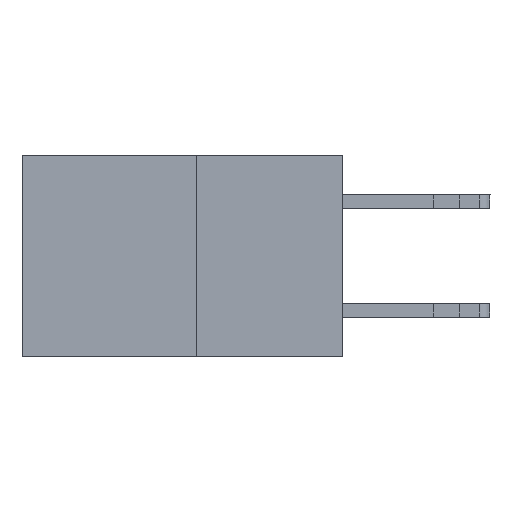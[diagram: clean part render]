
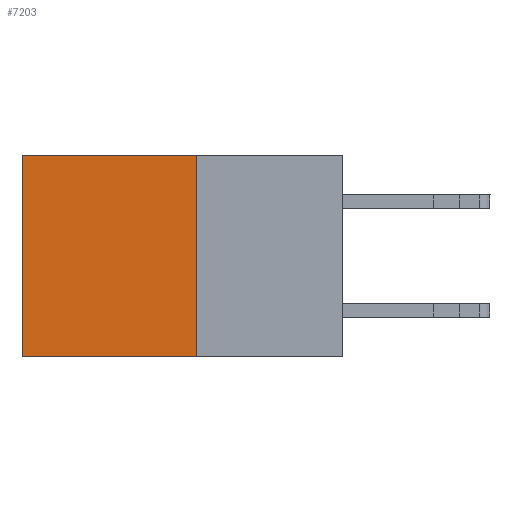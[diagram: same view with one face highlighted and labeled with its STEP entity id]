
A CAD part, left-side view. The second image highlights one B-rep face of the part: STEP entity #7203.
In plain terms, the highlighted planar face has unit normal (-1, 0, 0).
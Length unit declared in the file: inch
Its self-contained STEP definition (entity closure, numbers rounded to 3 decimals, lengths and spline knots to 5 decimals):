
#1 = VECTOR ( 'NONE', #10991, 39.37008 ) ;
#1696 = ORIENTED_EDGE ( 'NONE', *, *, #7137, .T. ) ;
#1968 = FACE_OUTER_BOUND ( 'NONE', #6050, .T. ) ;
#2018 = ORIENTED_EDGE ( 'NONE', *, *, #11326, .F. ) ;
#2251 = VERTEX_POINT ( 'NONE', #2997 ) ;
#2288 = VECTOR ( 'NONE', #6027, 39.37008 ) ;
#2997 = CARTESIAN_POINT ( 'NONE',  ( 0.277, 0.27, -0.37 ) ) ;
#4152 = VERTEX_POINT ( 'NONE', #9362 ) ;
#4315 = CARTESIAN_POINT ( 'NONE',  ( 0.277, 0.27, 0. ) ) ;
#5833 = LINE ( 'NONE', #11762, #2288 ) ;
#6027 = DIRECTION ( 'NONE',  ( 0., 1., 0. ) ) ;
#6050 = EDGE_LOOP ( 'NONE', ( #12384, #2018, #8611, #1696 ) ) ;
#6642 = LINE ( 'NONE', #11061, #1 ) ;
#6974 = EDGE_CURVE ( 'NONE', #4152, #8397, #10709, .T. ) ;
#7137 = EDGE_CURVE ( 'NONE', #12748, #4152, #6642, .T. ) ;
#7203 = ADVANCED_FACE ( 'NONE', ( #1968 ), #9122, .F. ) ;
#7771 = VECTOR ( 'NONE', #11431, 39.37008 ) ;
#8397 = VERTEX_POINT ( 'NONE', #8627 ) ;
#8549 = VECTOR ( 'NONE', #14202, 39.37008 ) ;
#8611 = ORIENTED_EDGE ( 'NONE', *, *, #8908, .F. ) ;
#8627 = CARTESIAN_POINT ( 'NONE',  ( 0.277, 0.59, -0.37 ) ) ;
#8790 = DIRECTION ( 'NONE',  ( 0., 0., -1. ) ) ;
#8835 = DIRECTION ( 'NONE',  ( 1., 0., 0. ) ) ;
#8908 = EDGE_CURVE ( 'NONE', #12748, #2251, #11950, .T. ) ;
#9122 = PLANE ( 'NONE',  #13848 ) ;
#9260 = CARTESIAN_POINT ( 'NONE',  ( 0.277, 0.27, -0.37 ) ) ;
#9362 = CARTESIAN_POINT ( 'NONE',  ( 0.277, 0.59, 0. ) ) ;
#9498 = CARTESIAN_POINT ( 'NONE',  ( 0.277, 0.27, -0.37 ) ) ;
#10709 = LINE ( 'NONE', #12743, #7771 ) ;
#10991 = DIRECTION ( 'NONE',  ( 0., 1., 0. ) ) ;
#11061 = CARTESIAN_POINT ( 'NONE',  ( 0.277, 0.27, 0. ) ) ;
#11326 = EDGE_CURVE ( 'NONE', #2251, #8397, #5833, .T. ) ;
#11431 = DIRECTION ( 'NONE',  ( 0., 0., -1. ) ) ;
#11762 = CARTESIAN_POINT ( 'NONE',  ( 0.277, 0.27, -0.37 ) ) ;
#11950 = LINE ( 'NONE', #9498, #8549 ) ;
#12384 = ORIENTED_EDGE ( 'NONE', *, *, #6974, .T. ) ;
#12743 = CARTESIAN_POINT ( 'NONE',  ( 0.277, 0.59, -0.37 ) ) ;
#12748 = VERTEX_POINT ( 'NONE', #4315 ) ;
#13848 = AXIS2_PLACEMENT_3D ( 'NONE', #9260, #8835, #8790 ) ;
#14202 = DIRECTION ( 'NONE',  ( 0., 0., -1. ) ) ;
